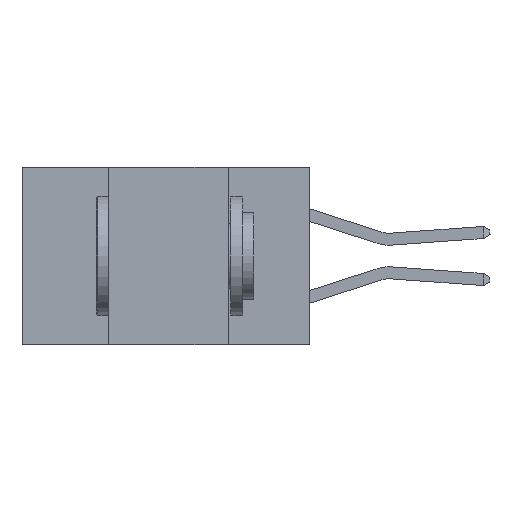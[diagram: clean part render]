
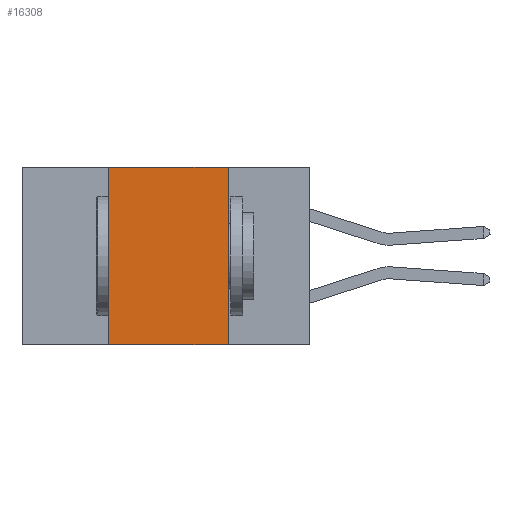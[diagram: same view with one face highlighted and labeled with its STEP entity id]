
A CAD part, left-side view. The second image highlights one B-rep face of the part: STEP entity #16308.
In plain terms, the highlighted planar face has unit normal (-1, 0, 0).
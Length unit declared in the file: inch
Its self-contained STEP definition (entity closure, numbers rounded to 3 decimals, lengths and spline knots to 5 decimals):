
#275 = EDGE_CURVE ( 'NONE', #8630, #13387, #4868, .T. ) ;
#628 = ORIENTED_EDGE ( 'NONE', *, *, #21995, .T. ) ;
#1009 = LINE ( 'NONE', #22159, #11451 ) ;
#1176 = EDGE_LOOP ( 'NONE', ( #17953, #3198, #9327, #628 ) ) ;
#1804 = VERTEX_POINT ( 'NONE', #8540 ) ;
#2430 = PLANE ( 'NONE',  #14717 ) ;
#2551 = DIRECTION ( 'NONE',  ( 1., 0., 0. ) ) ;
#3198 = ORIENTED_EDGE ( 'NONE', *, *, #12488, .F. ) ;
#3672 = DIRECTION ( 'NONE',  ( 0., 0., 1. ) ) ;
#4072 = CARTESIAN_POINT ( 'NONE',  ( 0., 0.6, 0. ) ) ;
#4619 = VERTEX_POINT ( 'NONE', #21749 ) ;
#4747 = CARTESIAN_POINT ( 'NONE',  ( 0., 0.17, -0.37 ) ) ;
#4868 = LINE ( 'NONE', #4747, #13833 ) ;
#5063 = CARTESIAN_POINT ( 'NONE',  ( 0., 0.17, 0. ) ) ;
#5559 = LINE ( 'NONE', #13256, #19411 ) ;
#8360 = FACE_OUTER_BOUND ( 'NONE', #1176, .T. ) ;
#8540 = CARTESIAN_POINT ( 'NONE',  ( 0., 0.42, -0.37 ) ) ;
#8630 = VERTEX_POINT ( 'NONE', #5063 ) ;
#9103 = VECTOR ( 'NONE', #16328, 39.37008 ) ;
#9327 = ORIENTED_EDGE ( 'NONE', *, *, #10083, .F. ) ;
#10083 = EDGE_CURVE ( 'NONE', #1804, #4619, #5559, .T. ) ;
#10968 = DIRECTION ( 'NONE',  ( 0., -1., 0. ) ) ;
#11451 = VECTOR ( 'NONE', #10968, 39.37008 ) ;
#12284 = CARTESIAN_POINT ( 'NONE',  ( 0., 0.6, -0.37 ) ) ;
#12488 = EDGE_CURVE ( 'NONE', #4619, #8630, #1009, .T. ) ;
#12561 = DIRECTION ( 'NONE',  ( 0., 0., -1. ) ) ;
#13256 = CARTESIAN_POINT ( 'NONE',  ( 0., 0.42, -0.37 ) ) ;
#13387 = VERTEX_POINT ( 'NONE', #22557 ) ;
#13833 = VECTOR ( 'NONE', #12561, 39.37008 ) ;
#14717 = AXIS2_PLACEMENT_3D ( 'NONE', #4072, #2551, #23458 ) ;
#16308 = ADVANCED_FACE ( 'NONE', ( #8360 ), #2430, .F. ) ;
#16328 = DIRECTION ( 'NONE',  ( 0., -1., 0. ) ) ;
#17953 = ORIENTED_EDGE ( 'NONE', *, *, #275, .F. ) ;
#19411 = VECTOR ( 'NONE', #3672, 39.37008 ) ;
#21749 = CARTESIAN_POINT ( 'NONE',  ( 0., 0.42, 0. ) ) ;
#21845 = LINE ( 'NONE', #12284, #9103 ) ;
#21995 = EDGE_CURVE ( 'NONE', #1804, #13387, #21845, .T. ) ;
#22159 = CARTESIAN_POINT ( 'NONE',  ( 0., 0.6, 0. ) ) ;
#22557 = CARTESIAN_POINT ( 'NONE',  ( 0., 0.17, -0.37 ) ) ;
#23458 = DIRECTION ( 'NONE',  ( 0., 0., -1. ) ) ;
